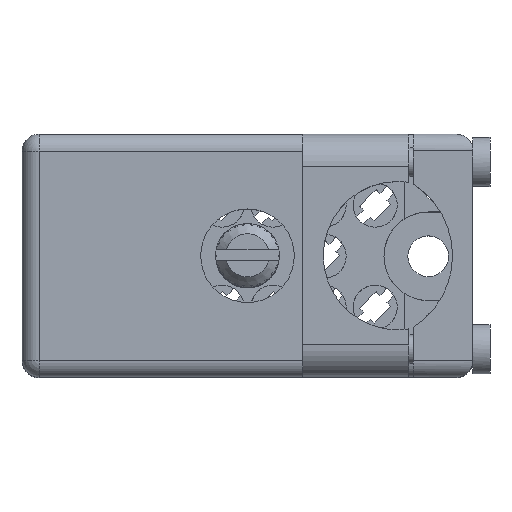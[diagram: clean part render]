
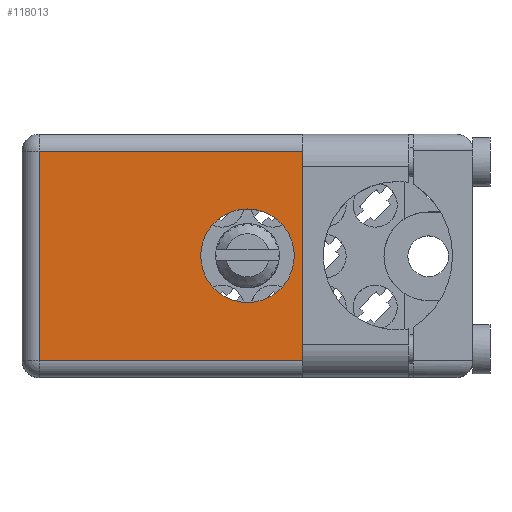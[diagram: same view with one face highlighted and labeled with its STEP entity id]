
A CAD part, top view. The second image highlights one B-rep face of the part: STEP entity #118013.
In plain terms, the highlighted face is planar.
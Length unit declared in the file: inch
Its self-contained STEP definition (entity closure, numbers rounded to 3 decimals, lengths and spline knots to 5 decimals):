
#13 = DIRECTION ( 'NONE',  ( 1., 0., 0. ) ) ;
#4010 = VECTOR ( 'NONE', #122021, 39.37008 ) ;
#4560 = LINE ( 'NONE', #154221, #154697 ) ;
#4936 = VERTEX_POINT ( 'NONE', #129485 ) ;
#9940 = EDGE_LOOP ( 'NONE', ( #30698, #96002 ) ) ;
#10281 = EDGE_CURVE ( 'NONE', #22789, #87667, #87640, .T. ) ;
#10697 = EDGE_CURVE ( 'NONE', #87667, #158474, #100810, .T. ) ;
#12467 = CARTESIAN_POINT ( 'NONE',  ( 0., 0.906, -0.715 ) ) ;
#14988 = CARTESIAN_POINT ( 'NONE',  ( 0.865, 0.906, -0.6025 ) ) ;
#22789 = VERTEX_POINT ( 'NONE', #144564 ) ;
#22980 = VERTEX_POINT ( 'NONE', #170804 ) ;
#23296 = CARTESIAN_POINT ( 'NONE',  ( 1.15, 0.906, -0.715 ) ) ;
#24691 = DIRECTION ( 'NONE',  ( -1., 0., 0. ) ) ;
#26173 = VERTEX_POINT ( 'NONE', #14988 ) ;
#26619 = DIRECTION ( 'NONE',  ( 0., 1., 0. ) ) ;
#27964 = DIRECTION ( 'NONE',  ( 0., 0., -1. ) ) ;
#28520 = CIRCLE ( 'NONE', #45642, 0.1375 ) ;
#30698 = ORIENTED_EDGE ( 'NONE', *, *, #87287, .F. ) ;
#32400 = ORIENTED_EDGE ( 'NONE', *, *, #75159, .T. ) ;
#36428 = CARTESIAN_POINT ( 'NONE',  ( 0., 0.906, -0.665 ) ) ;
#39955 = ORIENTED_EDGE ( 'NONE', *, *, #10281, .T. ) ;
#45642 = AXIS2_PLACEMENT_3D ( 'NONE', #91275, #149398, #62921 ) ;
#45916 = ORIENTED_EDGE ( 'NONE', *, *, #51194, .T. ) ;
#46130 = VERTEX_POINT ( 'NONE', #158938 ) ;
#46581 = VECTOR ( 'NONE', #24691, 39.37008 ) ;
#51194 = EDGE_CURVE ( 'NONE', #26173, #101010, #117621, .T. ) ;
#54179 = DIRECTION ( 'NONE',  ( -1., 0., 0. ) ) ;
#54194 = CARTESIAN_POINT ( 'NONE',  ( 0.05, 0.906, -0.05 ) ) ;
#54215 = EDGE_CURVE ( 'NONE', #69883, #4936, #4560, .T. ) ;
#55050 = CARTESIAN_POINT ( 'NONE',  ( 1.15, 0.906, -0.6025 ) ) ;
#58388 = DIRECTION ( 'NONE',  ( 0., 0., 1. ) ) ;
#62921 = DIRECTION ( 'NONE',  ( 0., 0., 1. ) ) ;
#64156 = EDGE_CURVE ( 'NONE', #69883, #158474, #154365, .T. ) ;
#66503 = ORIENTED_EDGE ( 'NONE', *, *, #150890, .F. ) ;
#69883 = VERTEX_POINT ( 'NONE', #122857 ) ;
#72707 = CARTESIAN_POINT ( 'NONE',  ( 1.15, 0.906, -0.665 ) ) ;
#75159 = EDGE_CURVE ( 'NONE', #133522, #22789, #97360, .T. ) ;
#77114 = CARTESIAN_POINT ( 'NONE',  ( 1.15, 0.906, -0.05 ) ) ;
#83201 = VECTOR ( 'NONE', #27964, 39.37008 ) ;
#83997 = CARTESIAN_POINT ( 'NONE',  ( 0.865, 0.906, -0.1125 ) ) ;
#86167 = CARTESIAN_POINT ( 'NONE',  ( 0.865, 0.906, -0.6025 ) ) ;
#87287 = EDGE_CURVE ( 'NONE', #22980, #46130, #28520, .T. ) ;
#87640 = LINE ( 'NONE', #168262, #182607 ) ;
#87667 = VERTEX_POINT ( 'NONE', #54194 ) ;
#91275 = CARTESIAN_POINT ( 'NONE',  ( 0.6625, 0.906, -0.3575 ) ) ;
#96002 = ORIENTED_EDGE ( 'NONE', *, *, #107972, .F. ) ;
#97360 = LINE ( 'NONE', #36428, #46581 ) ;
#97496 = DIRECTION ( 'NONE',  ( 0., 0., 1. ) ) ;
#100465 = EDGE_LOOP ( 'NONE', ( #39955, #130185, #108367, #134902, #110926, #45916, #66503, #32400 ) ) ;
#100810 = LINE ( 'NONE', #77114, #169367 ) ;
#101010 = VERTEX_POINT ( 'NONE', #55050 ) ;
#102195 = VECTOR ( 'NONE', #13, 39.37008 ) ;
#107972 = EDGE_CURVE ( 'NONE', #46130, #22980, #151805, .T. ) ;
#108367 = ORIENTED_EDGE ( 'NONE', *, *, #64156, .F. ) ;
#110926 = ORIENTED_EDGE ( 'NONE', *, *, #126351, .T. ) ;
#117621 = LINE ( 'NONE', #86167, #102195 ) ;
#118013 = ADVANCED_FACE ( 'NONE', ( #165941, #154995 ), #139568, .T. ) ;
#122021 = DIRECTION ( 'NONE',  ( 0., 0., 1. ) ) ;
#122326 = DIRECTION ( 'NONE',  ( 0., 1., 0. ) ) ;
#122857 = CARTESIAN_POINT ( 'NONE',  ( 1.15, 0.906, -0.1125 ) ) ;
#126351 = EDGE_CURVE ( 'NONE', #4936, #26173, #158403, .T. ) ;
#127565 = LINE ( 'NONE', #23296, #4010 ) ;
#129485 = CARTESIAN_POINT ( 'NONE',  ( 0.865, 0.906, -0.1125 ) ) ;
#130185 = ORIENTED_EDGE ( 'NONE', *, *, #10697, .T. ) ;
#133522 = VERTEX_POINT ( 'NONE', #72707 ) ;
#134902 = ORIENTED_EDGE ( 'NONE', *, *, #54215, .T. ) ;
#139568 = PLANE ( 'NONE',  #147640 ) ;
#141023 = CARTESIAN_POINT ( 'NONE',  ( 1.15, 0.906, -0.05 ) ) ;
#141076 = VECTOR ( 'NONE', #58388, 39.37008 ) ;
#141151 = DIRECTION ( 'NONE',  ( 0., 0., 1. ) ) ;
#143637 = CARTESIAN_POINT ( 'NONE',  ( 1.15, 0.906, -0.715 ) ) ;
#144564 = CARTESIAN_POINT ( 'NONE',  ( 0.05, 0.906, -0.665 ) ) ;
#147425 = AXIS2_PLACEMENT_3D ( 'NONE', #177803, #122326, #164315 ) ;
#147640 = AXIS2_PLACEMENT_3D ( 'NONE', #12467, #26619, #97496 ) ;
#149398 = DIRECTION ( 'NONE',  ( 0., 1., 0. ) ) ;
#150890 = EDGE_CURVE ( 'NONE', #133522, #101010, #127565, .T. ) ;
#151805 = CIRCLE ( 'NONE', #147425, 0.1375 ) ;
#154221 = CARTESIAN_POINT ( 'NONE',  ( 0.865, 0.906, -0.1125 ) ) ;
#154365 = LINE ( 'NONE', #143637, #141076 ) ;
#154697 = VECTOR ( 'NONE', #54179, 39.37008 ) ;
#154995 = FACE_BOUND ( 'NONE', #9940, .T. ) ;
#158403 = LINE ( 'NONE', #83997, #83201 ) ;
#158474 = VERTEX_POINT ( 'NONE', #141023 ) ;
#158938 = CARTESIAN_POINT ( 'NONE',  ( 0.6625, 0.906, -0.495 ) ) ;
#164315 = DIRECTION ( 'NONE',  ( 0., 0., 1. ) ) ;
#165941 = FACE_OUTER_BOUND ( 'NONE', #100465, .T. ) ;
#168262 = CARTESIAN_POINT ( 'NONE',  ( 0.05, 0.906, -0.715 ) ) ;
#169367 = VECTOR ( 'NONE', #175874, 39.37008 ) ;
#170804 = CARTESIAN_POINT ( 'NONE',  ( 0.6625, 0.906, -0.22 ) ) ;
#175874 = DIRECTION ( 'NONE',  ( 1., 0., 0. ) ) ;
#177803 = CARTESIAN_POINT ( 'NONE',  ( 0.6625, 0.906, -0.3575 ) ) ;
#182607 = VECTOR ( 'NONE', #141151, 39.37008 ) ;
